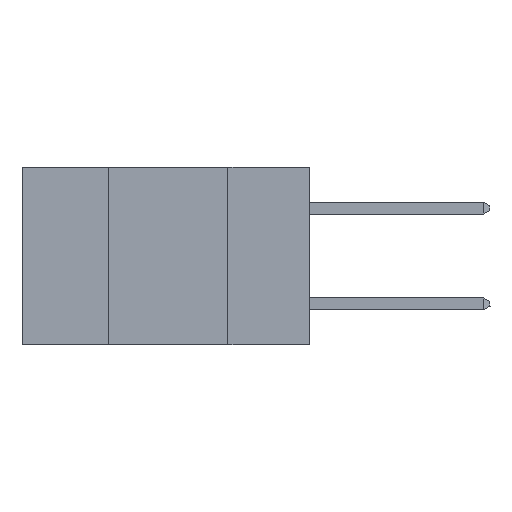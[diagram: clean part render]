
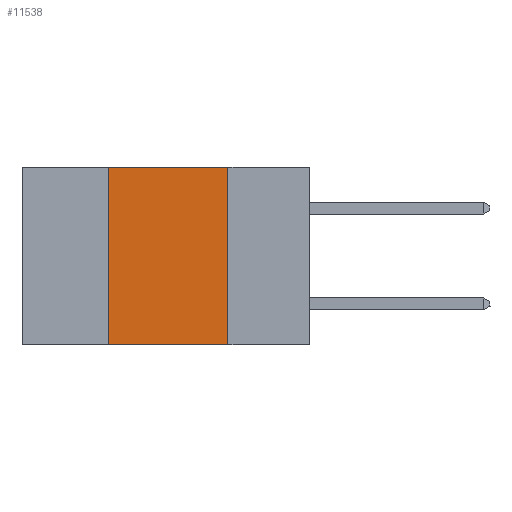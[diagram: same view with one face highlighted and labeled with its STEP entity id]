
A CAD part, left-side view. The second image highlights one B-rep face of the part: STEP entity #11538.
In plain terms, the highlighted planar face has unit normal (-1, 0, 0).
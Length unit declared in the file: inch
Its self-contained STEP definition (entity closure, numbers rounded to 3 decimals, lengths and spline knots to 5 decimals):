
#31 = CARTESIAN_POINT ( 'NONE',  ( 0., 0.17, -0.37 ) ) ;
#152 = VERTEX_POINT ( 'NONE', #1560 ) ;
#161 = VECTOR ( 'NONE', #11365, 39.37008 ) ;
#399 = CARTESIAN_POINT ( 'NONE',  ( 0., 0.6, -0.37 ) ) ;
#459 = VECTOR ( 'NONE', #11342, 39.37008 ) ;
#755 = CARTESIAN_POINT ( 'NONE',  ( 0., 0.6, 0. ) ) ;
#1016 = CARTESIAN_POINT ( 'NONE',  ( 0., 0.6, 0. ) ) ;
#1119 = CARTESIAN_POINT ( 'NONE',  ( 0., 0.17, 0. ) ) ;
#1560 = CARTESIAN_POINT ( 'NONE',  ( 0., 0.42, 0. ) ) ;
#1813 = PLANE ( 'NONE',  #9516 ) ;
#1886 = DIRECTION ( 'NONE',  ( 0., 0., -1. ) ) ;
#2943 = CARTESIAN_POINT ( 'NONE',  ( 0., 0.17, 0. ) ) ;
#3124 = ORIENTED_EDGE ( 'NONE', *, *, #6762, .F. ) ;
#3906 = ORIENTED_EDGE ( 'NONE', *, *, #8116, .F. ) ;
#6586 = LINE ( 'NONE', #2943, #13157 ) ;
#6748 = FACE_OUTER_BOUND ( 'NONE', #6998, .T. ) ;
#6762 = EDGE_CURVE ( 'NONE', #7004, #152, #12805, .T. ) ;
#6817 = DIRECTION ( 'NONE',  ( 0., 0., -1. ) ) ;
#6998 = EDGE_LOOP ( 'NONE', ( #13365, #3906, #3124, #15619 ) ) ;
#7004 = VERTEX_POINT ( 'NONE', #9818 ) ;
#7982 = VERTEX_POINT ( 'NONE', #1119 ) ;
#8116 = EDGE_CURVE ( 'NONE', #152, #7982, #9658, .T. ) ;
#9516 = AXIS2_PLACEMENT_3D ( 'NONE', #755, #12964, #1886 ) ;
#9658 = LINE ( 'NONE', #1016, #459 ) ;
#9818 = CARTESIAN_POINT ( 'NONE',  ( 0., 0.42, -0.37 ) ) ;
#10212 = EDGE_CURVE ( 'NONE', #7982, #11859, #6586, .T. ) ;
#11342 = DIRECTION ( 'NONE',  ( 0., -1., 0. ) ) ;
#11365 = DIRECTION ( 'NONE',  ( 0., 0., 1. ) ) ;
#11463 = VECTOR ( 'NONE', #14072, 39.37008 ) ;
#11538 = ADVANCED_FACE ( 'NONE', ( #6748 ), #1813, .F. ) ;
#11859 = VERTEX_POINT ( 'NONE', #31 ) ;
#12693 = LINE ( 'NONE', #399, #11463 ) ;
#12805 = LINE ( 'NONE', #12883, #161 ) ;
#12883 = CARTESIAN_POINT ( 'NONE',  ( 0., 0.42, 0. ) ) ;
#12964 = DIRECTION ( 'NONE',  ( 1., 0., 0. ) ) ;
#13157 = VECTOR ( 'NONE', #6817, 39.37008 ) ;
#13365 = ORIENTED_EDGE ( 'NONE', *, *, #10212, .F. ) ;
#14072 = DIRECTION ( 'NONE',  ( 0., -1., 0. ) ) ;
#14618 = EDGE_CURVE ( 'NONE', #7004, #11859, #12693, .T. ) ;
#15619 = ORIENTED_EDGE ( 'NONE', *, *, #14618, .T. ) ;
